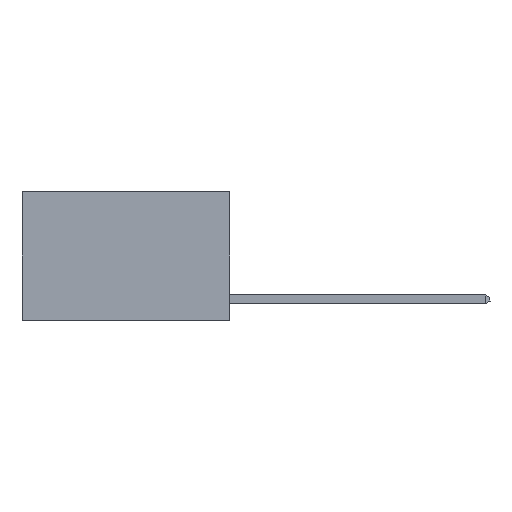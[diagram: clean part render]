
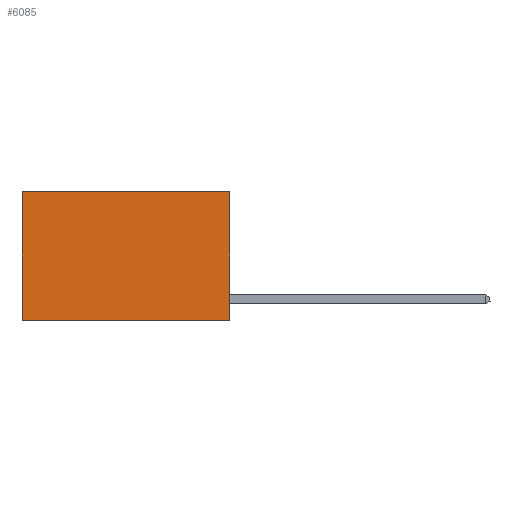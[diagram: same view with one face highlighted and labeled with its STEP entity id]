
A CAD part, left-side view. The second image highlights one B-rep face of the part: STEP entity #6085.
In plain terms, the highlighted planar face has unit normal (-1, 0, 0).
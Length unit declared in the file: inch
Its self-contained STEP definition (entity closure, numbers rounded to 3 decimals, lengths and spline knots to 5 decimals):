
#43 = CARTESIAN_POINT ( 'NONE',  ( 0.2625, 0., 0. ) ) ;
#88 = FACE_OUTER_BOUND ( 'NONE', #8001, .T. ) ;
#99 = VERTEX_POINT ( 'NONE', #5693 ) ;
#164 = VECTOR ( 'NONE', #4654, 39.37008 ) ;
#882 = VERTEX_POINT ( 'NONE', #2538 ) ;
#1322 = CARTESIAN_POINT ( 'NONE',  ( 0.2625, 0., 0. ) ) ;
#2129 = DIRECTION ( 'NONE',  ( 0., 1., 0. ) ) ;
#2338 = DIRECTION ( 'NONE',  ( 0., 0., -1. ) ) ;
#2420 = EDGE_CURVE ( 'NONE', #882, #99, #5548, .T. ) ;
#2515 = ORIENTED_EDGE ( 'NONE', *, *, #4899, .T. ) ;
#2538 = CARTESIAN_POINT ( 'NONE',  ( 0.2625, 0., -0.37 ) ) ;
#2625 = EDGE_CURVE ( 'NONE', #8123, #882, #5603, .T. ) ;
#2856 = VECTOR ( 'NONE', #2129, 39.37008 ) ;
#3036 = CARTESIAN_POINT ( 'NONE',  ( 0.2625, 0., 0. ) ) ;
#3611 = DIRECTION ( 'NONE',  ( 0., 0., -1. ) ) ;
#3983 = VERTEX_POINT ( 'NONE', #4988 ) ;
#4263 = ORIENTED_EDGE ( 'NONE', *, *, #2625, .F. ) ;
#4492 = VECTOR ( 'NONE', #2338, 39.37008 ) ;
#4654 = DIRECTION ( 'NONE',  ( 0., 1., 0. ) ) ;
#4899 = EDGE_CURVE ( 'NONE', #8123, #3983, #6520, .T. ) ;
#4988 = CARTESIAN_POINT ( 'NONE',  ( 0.2625, 0.6, 0. ) ) ;
#5455 = PLANE ( 'NONE',  #8306 ) ;
#5542 = DIRECTION ( 'NONE',  ( 0., 0., -1. ) ) ;
#5548 = LINE ( 'NONE', #6932, #2856 ) ;
#5603 = LINE ( 'NONE', #3036, #6980 ) ;
#5693 = CARTESIAN_POINT ( 'NONE',  ( 0.2625, 0.6, -0.37 ) ) ;
#6085 = ADVANCED_FACE ( 'NONE', ( #88 ), #5455, .F. ) ;
#6275 = ORIENTED_EDGE ( 'NONE', *, *, #6540, .T. ) ;
#6520 = LINE ( 'NONE', #1322, #164 ) ;
#6540 = EDGE_CURVE ( 'NONE', #3983, #99, #7096, .T. ) ;
#6932 = CARTESIAN_POINT ( 'NONE',  ( 0.2625, 0., -0.37 ) ) ;
#6980 = VECTOR ( 'NONE', #3611, 39.37008 ) ;
#7051 = CARTESIAN_POINT ( 'NONE',  ( 0.2625, 0.6, 0. ) ) ;
#7096 = LINE ( 'NONE', #7051, #4492 ) ;
#7501 = DIRECTION ( 'NONE',  ( 1., 0., 0. ) ) ;
#8001 = EDGE_LOOP ( 'NONE', ( #6275, #8756, #4263, #2515 ) ) ;
#8123 = VERTEX_POINT ( 'NONE', #8273 ) ;
#8273 = CARTESIAN_POINT ( 'NONE',  ( 0.2625, 0., 0. ) ) ;
#8306 = AXIS2_PLACEMENT_3D ( 'NONE', #43, #7501, #5542 ) ;
#8756 = ORIENTED_EDGE ( 'NONE', *, *, #2420, .F. ) ;
